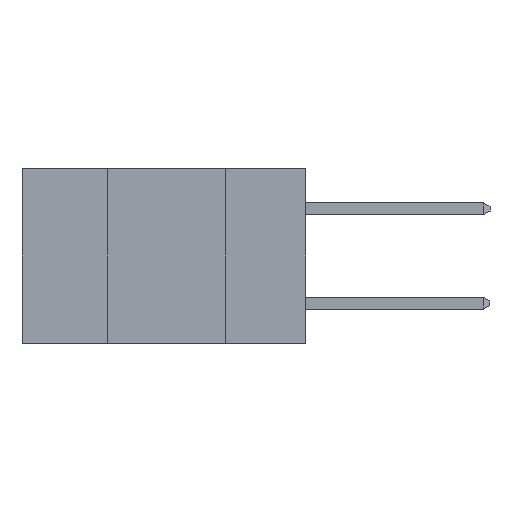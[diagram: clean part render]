
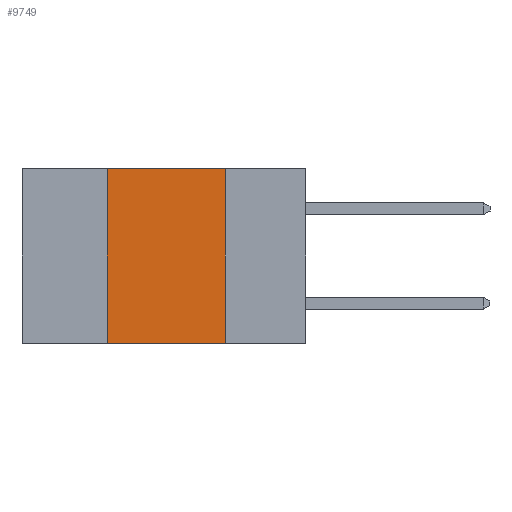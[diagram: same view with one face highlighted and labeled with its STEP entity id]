
A CAD part, left-side view. The second image highlights one B-rep face of the part: STEP entity #9749.
In plain terms, the highlighted planar face has unit normal (-1, 0, 0).
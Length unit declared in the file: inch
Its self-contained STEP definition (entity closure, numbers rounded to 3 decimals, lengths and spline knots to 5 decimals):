
#534 = DIRECTION ( 'NONE',  ( 0., 0., -1. ) ) ;
#548 = DIRECTION ( 'NONE',  ( 1., 0., 0. ) ) ;
#553 = CARTESIAN_POINT ( 'NONE',  ( 0., 0.6, 0. ) ) ;
#696 = PLANE ( 'NONE',  #8899 ) ;
#1756 = LINE ( 'NONE', #8131, #4640 ) ;
#2361 = CARTESIAN_POINT ( 'NONE',  ( 0., 0.17, 0. ) ) ;
#3733 = CARTESIAN_POINT ( 'NONE',  ( 0., 0.17, -0.37 ) ) ;
#4191 = EDGE_CURVE ( 'NONE', #7230, #13457, #7006, .T. ) ;
#4566 = DIRECTION ( 'NONE',  ( 0., -1., 0. ) ) ;
#4640 = VECTOR ( 'NONE', #7809, 39.37008 ) ;
#4773 = ORIENTED_EDGE ( 'NONE', *, *, #4191, .F. ) ;
#5383 = CARTESIAN_POINT ( 'NONE',  ( 0., 0.42, 0. ) ) ;
#7006 = LINE ( 'NONE', #8234, #13079 ) ;
#7066 = CARTESIAN_POINT ( 'NONE',  ( 0., 0.17, 0. ) ) ;
#7230 = VERTEX_POINT ( 'NONE', #8919 ) ;
#7238 = DIRECTION ( 'NONE',  ( 0., 0., -1. ) ) ;
#7245 = ORIENTED_EDGE ( 'NONE', *, *, #8858, .F. ) ;
#7272 = EDGE_CURVE ( 'NONE', #13457, #11707, #1756, .T. ) ;
#7669 = VECTOR ( 'NONE', #7238, 39.37008 ) ;
#7809 = DIRECTION ( 'NONE',  ( 0., -1., 0. ) ) ;
#8131 = CARTESIAN_POINT ( 'NONE',  ( 0., 0.6, 0. ) ) ;
#8234 = CARTESIAN_POINT ( 'NONE',  ( 0., 0.42, 0. ) ) ;
#8858 = EDGE_CURVE ( 'NONE', #11707, #15139, #10860, .T. ) ;
#8899 = AXIS2_PLACEMENT_3D ( 'NONE', #553, #548, #534 ) ;
#8919 = CARTESIAN_POINT ( 'NONE',  ( 0., 0.42, -0.37 ) ) ;
#9749 = ADVANCED_FACE ( 'NONE', ( #10587 ), #696, .F. ) ;
#10091 = VECTOR ( 'NONE', #4566, 39.37008 ) ;
#10587 = FACE_OUTER_BOUND ( 'NONE', #12227, .T. ) ;
#10860 = LINE ( 'NONE', #7066, #7669 ) ;
#11707 = VERTEX_POINT ( 'NONE', #2361 ) ;
#12227 = EDGE_LOOP ( 'NONE', ( #7245, #14083, #4773, #14445 ) ) ;
#13079 = VECTOR ( 'NONE', #14783, 39.37008 ) ;
#13273 = LINE ( 'NONE', #14282, #10091 ) ;
#13457 = VERTEX_POINT ( 'NONE', #5383 ) ;
#14083 = ORIENTED_EDGE ( 'NONE', *, *, #7272, .F. ) ;
#14265 = EDGE_CURVE ( 'NONE', #7230, #15139, #13273, .T. ) ;
#14282 = CARTESIAN_POINT ( 'NONE',  ( 0., 0.6, -0.37 ) ) ;
#14445 = ORIENTED_EDGE ( 'NONE', *, *, #14265, .T. ) ;
#14783 = DIRECTION ( 'NONE',  ( 0., 0., 1. ) ) ;
#15139 = VERTEX_POINT ( 'NONE', #3733 ) ;
